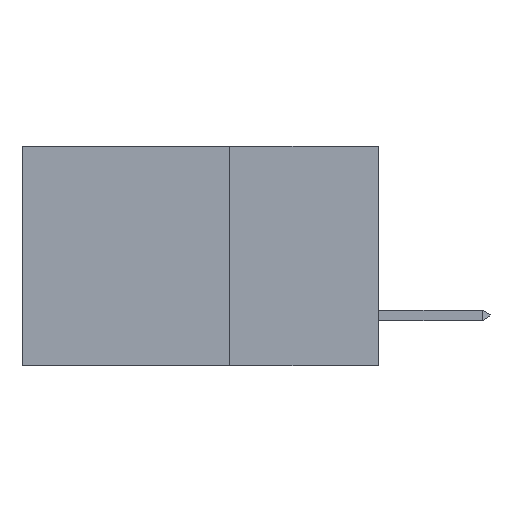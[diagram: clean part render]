
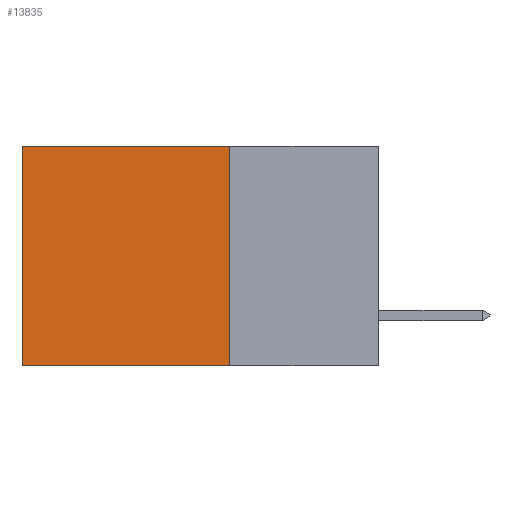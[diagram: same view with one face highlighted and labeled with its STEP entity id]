
A CAD part, left-side view. The second image highlights one B-rep face of the part: STEP entity #13835.
In plain terms, the highlighted planar face has unit normal (-1, 0, 0).
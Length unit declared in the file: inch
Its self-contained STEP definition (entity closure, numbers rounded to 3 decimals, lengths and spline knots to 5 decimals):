
#313 = EDGE_CURVE ( 'NONE', #18989, #26711, #14175, .T. ) ;
#1068 = LINE ( 'NONE', #13349, #5435 ) ;
#1816 = ORIENTED_EDGE ( 'NONE', *, *, #9432, .F. ) ;
#3511 = LINE ( 'NONE', #17958, #27505 ) ;
#3689 = DIRECTION ( 'NONE',  ( 0., 0., -1. ) ) ;
#4695 = AXIS2_PLACEMENT_3D ( 'NONE', #12679, #21996, #19954 ) ;
#5435 = VECTOR ( 'NONE', #17798, 39.37008 ) ;
#6470 = VECTOR ( 'NONE', #26490, 39.37008 ) ;
#9432 = EDGE_CURVE ( 'NONE', #16227, #10659, #3511, .T. ) ;
#10659 = VERTEX_POINT ( 'NONE', #22617 ) ;
#12679 = CARTESIAN_POINT ( 'NONE',  ( 0.298, 0.25, 0. ) ) ;
#12727 = VECTOR ( 'NONE', #26210, 39.37008 ) ;
#13349 = CARTESIAN_POINT ( 'NONE',  ( 0.298, 0.25, 0. ) ) ;
#13384 = ORIENTED_EDGE ( 'NONE', *, *, #17036, .F. ) ;
#13835 = ADVANCED_FACE ( 'NONE', ( #29803 ), #17530, .F. ) ;
#14175 = LINE ( 'NONE', #14486, #12727 ) ;
#14486 = CARTESIAN_POINT ( 'NONE',  ( 0.298, 0.6, 0. ) ) ;
#14497 = ORIENTED_EDGE ( 'NONE', *, *, #313, .T. ) ;
#14506 = LINE ( 'NONE', #26389, #6470 ) ;
#16227 = VERTEX_POINT ( 'NONE', #29938 ) ;
#17036 = EDGE_CURVE ( 'NONE', #10659, #26711, #14506, .T. ) ;
#17530 = PLANE ( 'NONE',  #4695 ) ;
#17798 = DIRECTION ( 'NONE',  ( 0., 1., 0. ) ) ;
#17958 = CARTESIAN_POINT ( 'NONE',  ( 0.298, 0.25, 0. ) ) ;
#18989 = VERTEX_POINT ( 'NONE', #24171 ) ;
#19954 = DIRECTION ( 'NONE',  ( 0., 0., -1. ) ) ;
#21996 = DIRECTION ( 'NONE',  ( 1., 0., 0. ) ) ;
#22617 = CARTESIAN_POINT ( 'NONE',  ( 0.298, 0.25, -0.37 ) ) ;
#22936 = EDGE_LOOP ( 'NONE', ( #14497, #13384, #1816, #23789 ) ) ;
#23789 = ORIENTED_EDGE ( 'NONE', *, *, #29480, .T. ) ;
#24171 = CARTESIAN_POINT ( 'NONE',  ( 0.298, 0.6, 0. ) ) ;
#26210 = DIRECTION ( 'NONE',  ( 0., 0., -1. ) ) ;
#26389 = CARTESIAN_POINT ( 'NONE',  ( 0.298, 0.25, -0.37 ) ) ;
#26490 = DIRECTION ( 'NONE',  ( 0., 1., 0. ) ) ;
#26711 = VERTEX_POINT ( 'NONE', #28627 ) ;
#27505 = VECTOR ( 'NONE', #3689, 39.37008 ) ;
#28627 = CARTESIAN_POINT ( 'NONE',  ( 0.298, 0.6, -0.37 ) ) ;
#29480 = EDGE_CURVE ( 'NONE', #16227, #18989, #1068, .T. ) ;
#29803 = FACE_OUTER_BOUND ( 'NONE', #22936, .T. ) ;
#29938 = CARTESIAN_POINT ( 'NONE',  ( 0.298, 0.25, 0. ) ) ;
